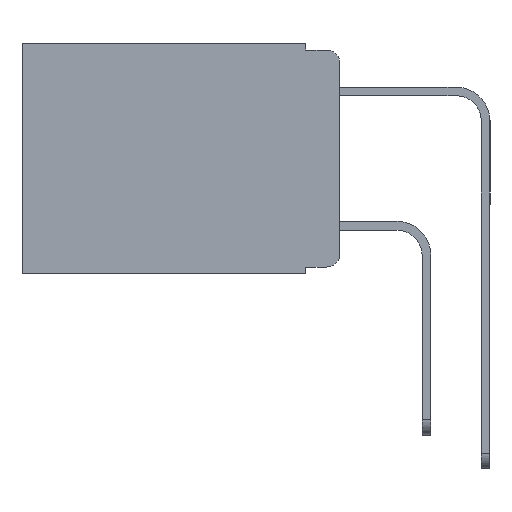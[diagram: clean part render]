
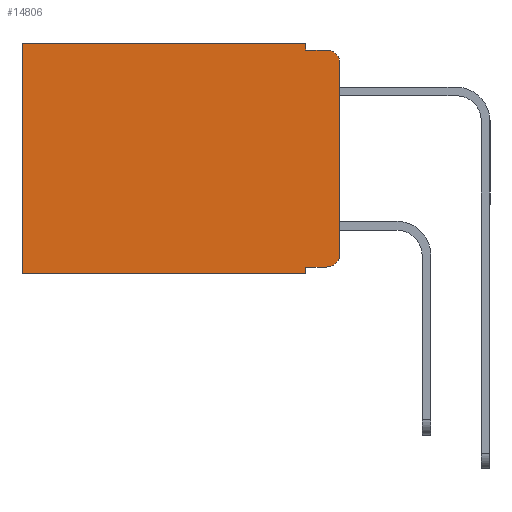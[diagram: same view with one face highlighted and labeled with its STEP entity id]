
A CAD part, left-side view. The second image highlights one B-rep face of the part: STEP entity #14806.
In plain terms, the highlighted planar face has unit normal (-1, 0, 0).
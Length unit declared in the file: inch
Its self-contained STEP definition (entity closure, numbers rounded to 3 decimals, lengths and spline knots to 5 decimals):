
#54 = EDGE_CURVE ( 'NONE', #3985, #11456, #3647, .T. ) ;
#277 = VECTOR ( 'NONE', #8462, 39.37008 ) ;
#375 = VECTOR ( 'NONE', #8786, 39.37008 ) ;
#427 = VECTOR ( 'NONE', #14976, 39.37008 ) ;
#771 = CARTESIAN_POINT ( 'NONE',  ( 0.298, 0.473, -0.343 ) ) ;
#976 = CARTESIAN_POINT ( 'NONE',  ( 0.298, 0., -0.343 ) ) ;
#1230 = CARTESIAN_POINT ( 'NONE',  ( 0.298, 0., 0. ) ) ;
#1234 = VERTEX_POINT ( 'NONE', #9791 ) ;
#1329 = ORIENTED_EDGE ( 'NONE', *, *, #6498, .T. ) ;
#1664 = VECTOR ( 'NONE', #4825, 39.37008 ) ;
#1747 = VERTEX_POINT ( 'NONE', #5015 ) ;
#1952 = VECTOR ( 'NONE', #14627, 39.37008 ) ;
#2107 = VERTEX_POINT ( 'NONE', #7265 ) ;
#2438 = VERTEX_POINT ( 'NONE', #771 ) ;
#2752 = LINE ( 'NONE', #1230, #1952 ) ;
#2840 = CARTESIAN_POINT ( 'NONE',  ( 0.298, 0.02, -0.03 ) ) ;
#2904 = EDGE_CURVE ( 'NONE', #2107, #8306, #2752, .T. ) ;
#3488 = LINE ( 'NONE', #14598, #4648 ) ;
#3647 = LINE ( 'NONE', #10440, #277 ) ;
#3804 = ORIENTED_EDGE ( 'NONE', *, *, #11441, .F. ) ;
#3860 = PLANE ( 'NONE',  #15427 ) ;
#3956 = EDGE_CURVE ( 'NONE', #1747, #8306, #4095, .T. ) ;
#3985 = VERTEX_POINT ( 'NONE', #4845 ) ;
#3997 = CARTESIAN_POINT ( 'NONE',  ( 0.298, 0.473, 0. ) ) ;
#4087 = DIRECTION ( 'NONE',  ( 0., 0., -1. ) ) ;
#4095 = CIRCLE ( 'NONE', #10134, 0.02 ) ;
#4112 = LINE ( 'NONE', #9905, #375 ) ;
#4397 = ORIENTED_EDGE ( 'NONE', *, *, #12745, .T. ) ;
#4648 = VECTOR ( 'NONE', #6078, 39.37008 ) ;
#4825 = DIRECTION ( 'NONE',  ( 0., 1., 0. ) ) ;
#4845 = CARTESIAN_POINT ( 'NONE',  ( 0.298, 0.051, -0.01 ) ) ;
#5004 = LINE ( 'NONE', #976, #1664 ) ;
#5015 = CARTESIAN_POINT ( 'NONE',  ( 0.298, 0.02, -0.333 ) ) ;
#5750 = DIRECTION ( 'NONE',  ( 0., 1., 0. ) ) ;
#5816 = DIRECTION ( 'NONE',  ( 0., 0., -1. ) ) ;
#6078 = DIRECTION ( 'NONE',  ( 0., -1., 0. ) ) ;
#6298 = CARTESIAN_POINT ( 'NONE',  ( 0.298, 0., 0. ) ) ;
#6498 = EDGE_CURVE ( 'NONE', #9741, #2438, #9916, .T. ) ;
#7247 = CARTESIAN_POINT ( 'NONE',  ( 0.298, 0.02, -0.313 ) ) ;
#7265 = CARTESIAN_POINT ( 'NONE',  ( 0.298, 0., -0.03 ) ) ;
#7564 = DIRECTION ( 'NONE',  ( 0., 0., -1. ) ) ;
#7867 = VERTEX_POINT ( 'NONE', #10282 ) ;
#7932 = ORIENTED_EDGE ( 'NONE', *, *, #9808, .T. ) ;
#8019 = ORIENTED_EDGE ( 'NONE', *, *, #2904, .F. ) ;
#8198 = CARTESIAN_POINT ( 'NONE',  ( 0.298, 0., 0. ) ) ;
#8306 = VERTEX_POINT ( 'NONE', #13565 ) ;
#8462 = DIRECTION ( 'NONE',  ( 0., -1., 0. ) ) ;
#8507 = DIRECTION ( 'NONE',  ( 0., 0., -1. ) ) ;
#8786 = DIRECTION ( 'NONE',  ( 0., 0., -1. ) ) ;
#9741 = VERTEX_POINT ( 'NONE', #13293 ) ;
#9770 = VECTOR ( 'NONE', #5750, 39.37008 ) ;
#9791 = CARTESIAN_POINT ( 'NONE',  ( 0.298, 0.051, 0. ) ) ;
#9808 = EDGE_CURVE ( 'NONE', #12809, #1747, #3488, .T. ) ;
#9905 = CARTESIAN_POINT ( 'NONE',  ( 0.298, 0.051, 0. ) ) ;
#9916 = LINE ( 'NONE', #3997, #427 ) ;
#10134 = AXIS2_PLACEMENT_3D ( 'NONE', #7247, #15723, #8507 ) ;
#10140 = ORIENTED_EDGE ( 'NONE', *, *, #54, .F. ) ;
#10282 = CARTESIAN_POINT ( 'NONE',  ( 0.298, 0.051, -0.343 ) ) ;
#10440 = CARTESIAN_POINT ( 'NONE',  ( 0.298, 0.051, -0.01 ) ) ;
#10575 = FACE_OUTER_BOUND ( 'NONE', #13331, .T. ) ;
#10869 = AXIS2_PLACEMENT_3D ( 'NONE', #2840, #11427, #4087 ) ;
#10997 = ORIENTED_EDGE ( 'NONE', *, *, #3956, .T. ) ;
#11427 = DIRECTION ( 'NONE',  ( -1., 0., 0. ) ) ;
#11441 = EDGE_CURVE ( 'NONE', #1234, #3985, #12920, .T. ) ;
#11456 = VERTEX_POINT ( 'NONE', #14389 ) ;
#12060 = EDGE_CURVE ( 'NONE', #12809, #7867, #4112, .T. ) ;
#12745 = EDGE_CURVE ( 'NONE', #2107, #11456, #14954, .T. ) ;
#12809 = VERTEX_POINT ( 'NONE', #15157 ) ;
#12824 = ORIENTED_EDGE ( 'NONE', *, *, #14289, .F. ) ;
#12920 = LINE ( 'NONE', #15543, #15750 ) ;
#12986 = LINE ( 'NONE', #8198, #9770 ) ;
#13238 = ORIENTED_EDGE ( 'NONE', *, *, #15776, .T. ) ;
#13293 = CARTESIAN_POINT ( 'NONE',  ( 0.298, 0.473, 0. ) ) ;
#13331 = EDGE_LOOP ( 'NONE', ( #8019, #4397, #10140, #3804, #13238, #1329, #12824, #15535, #7932, #10997 ) ) ;
#13565 = CARTESIAN_POINT ( 'NONE',  ( 0.298, 0., -0.313 ) ) ;
#14289 = EDGE_CURVE ( 'NONE', #7867, #2438, #5004, .T. ) ;
#14389 = CARTESIAN_POINT ( 'NONE',  ( 0.298, 0.02, -0.01 ) ) ;
#14598 = CARTESIAN_POINT ( 'NONE',  ( 0.298, 0.051, -0.333 ) ) ;
#14627 = DIRECTION ( 'NONE',  ( 0., 0., -1. ) ) ;
#14806 = ADVANCED_FACE ( 'NONE', ( #10575 ), #3860, .F. ) ;
#14832 = DIRECTION ( 'NONE',  ( 1., 0., 0. ) ) ;
#14954 = CIRCLE ( 'NONE', #10869, 0.02 ) ;
#14976 = DIRECTION ( 'NONE',  ( 0., 0., -1. ) ) ;
#15157 = CARTESIAN_POINT ( 'NONE',  ( 0.298, 0.051, -0.333 ) ) ;
#15427 = AXIS2_PLACEMENT_3D ( 'NONE', #6298, #14832, #7564 ) ;
#15535 = ORIENTED_EDGE ( 'NONE', *, *, #12060, .F. ) ;
#15543 = CARTESIAN_POINT ( 'NONE',  ( 0.298, 0.051, 0. ) ) ;
#15723 = DIRECTION ( 'NONE',  ( -1., 0., 0. ) ) ;
#15750 = VECTOR ( 'NONE', #5816, 39.37008 ) ;
#15776 = EDGE_CURVE ( 'NONE', #1234, #9741, #12986, .T. ) ;
